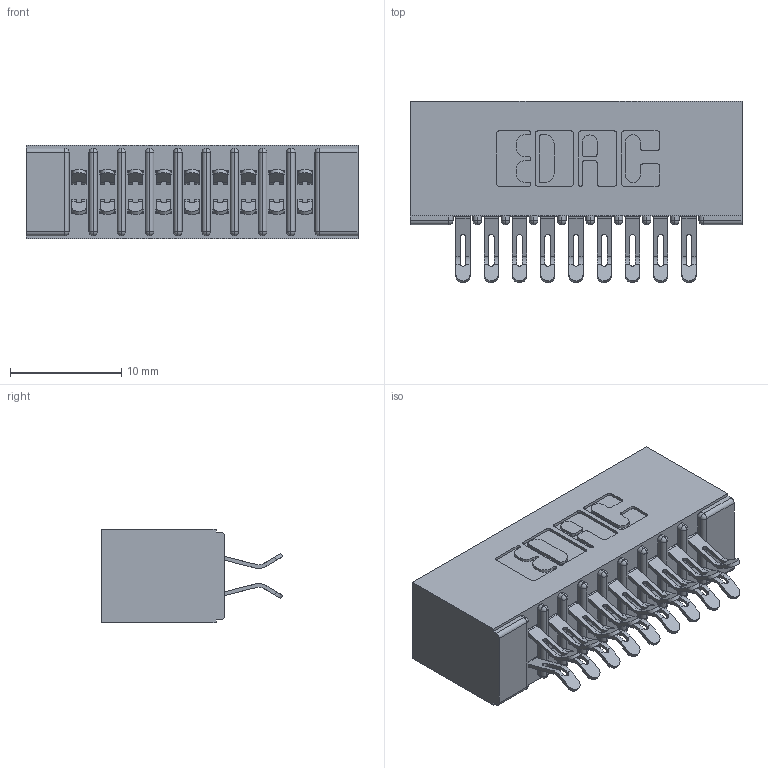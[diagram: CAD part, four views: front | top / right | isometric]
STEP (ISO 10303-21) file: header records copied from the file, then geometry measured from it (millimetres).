
FILE_DESCRIPTION (( 'STEP AP203' ), '1' );
FILE_NAME ('341-018-555-201.STEP', '2018-08-06T16:20:42', ( '' ), ( '' ), 'SwSTEP 2.0', 'SolidWorks 2016', '' );
FILE_SCHEMA (( 'CONFIG_CONTROL_DESIGN' ));
Length unit declared in the file: inch
Products named in the file (3): 341-018-555-201; 341 Part_No Mounting Lugs; 341-292-001_341-292-155
Assembly tree (19 placements, depth 2):
  341-018-555-201
    341 Part_No Mounting Lugs
    341-292-001_341-292-155  x18
Bounding box: 29.84 x 16.31 x 8.38 mm (x, y, z)
Volume: 1886.3 mm3; surface area: 3944.3 mm2
Topology: 19 solids, 19 shells, 1512 faces, 4495 edges, 2926 vertices
Faces by surface type: plane 820, cylinder 656, sphere 20, torus 16
Entity records: 15480 total; most frequent: CARTESIAN_POINT 2589, ORIENTED_EDGE 2558, DIRECTION 2525, EDGE_CURVE 1279, LINE 985, VECTOR 985, VERTEX_POINT 818, AXIS2_PLACEMENT_3D 770
